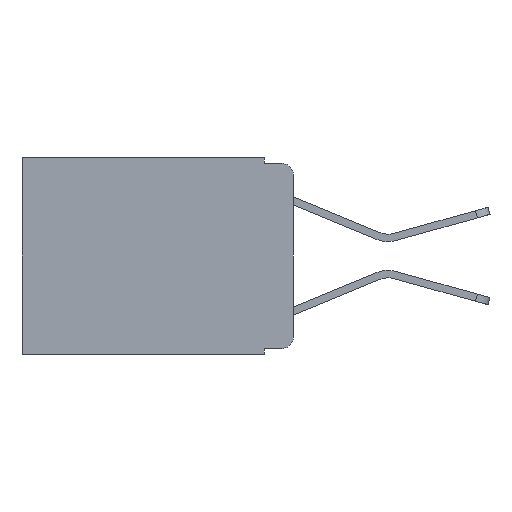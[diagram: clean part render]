
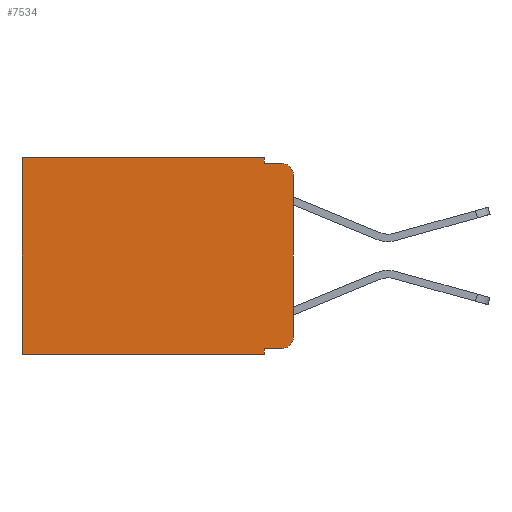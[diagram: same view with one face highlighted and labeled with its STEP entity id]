
A CAD part, left-side view. The second image highlights one B-rep face of the part: STEP entity #7534.
In plain terms, the highlighted planar face has unit normal (-1, 0, 0).
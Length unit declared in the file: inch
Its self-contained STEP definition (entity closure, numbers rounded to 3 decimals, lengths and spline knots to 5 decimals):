
#37 = DIRECTION ( 'NONE',  ( 0., 1., 0. ) ) ;
#145 = PLANE ( 'NONE',  #11362 ) ;
#223 = CARTESIAN_POINT ( 'NONE',  ( 0.298, 0.051, -0.333 ) ) ;
#269 = VERTEX_POINT ( 'NONE', #6955 ) ;
#425 = CARTESIAN_POINT ( 'NONE',  ( 0.298, 0.051, 0. ) ) ;
#492 = VERTEX_POINT ( 'NONE', #12710 ) ;
#496 = VERTEX_POINT ( 'NONE', #12790 ) ;
#734 = VECTOR ( 'NONE', #9410, 39.37008 ) ;
#867 = ORIENTED_EDGE ( 'NONE', *, *, #4749, .T. ) ;
#1336 = LINE ( 'NONE', #6577, #9643 ) ;
#1829 = DIRECTION ( 'NONE',  ( 0., 0., -1. ) ) ;
#1832 = CIRCLE ( 'NONE', #12632, 0.02 ) ;
#1895 = VERTEX_POINT ( 'NONE', #7905 ) ;
#1909 = VERTEX_POINT ( 'NONE', #4972 ) ;
#1985 = DIRECTION ( 'NONE',  ( 0., 0., -1. ) ) ;
#2217 = EDGE_CURVE ( 'NONE', #269, #6151, #1832, .T. ) ;
#2227 = ORIENTED_EDGE ( 'NONE', *, *, #4703, .F. ) ;
#2399 = EDGE_CURVE ( 'NONE', #11240, #269, #12608, .T. ) ;
#2665 = DIRECTION ( 'NONE',  ( 0., 0., -1. ) ) ;
#2772 = CARTESIAN_POINT ( 'NONE',  ( 0.298, 0., -0.03 ) ) ;
#3030 = CARTESIAN_POINT ( 'NONE',  ( 0.298, 0.051, -0.01 ) ) ;
#3244 = CIRCLE ( 'NONE', #12895, 0.02 ) ;
#4007 = ORIENTED_EDGE ( 'NONE', *, *, #4654, .F. ) ;
#4210 = DIRECTION ( 'NONE',  ( 0., -1., 0. ) ) ;
#4489 = LINE ( 'NONE', #11595, #9788 ) ;
#4553 = EDGE_CURVE ( 'NONE', #7193, #6151, #9804, .T. ) ;
#4568 = ORIENTED_EDGE ( 'NONE', *, *, #4945, .F. ) ;
#4598 = EDGE_CURVE ( 'NONE', #7193, #492, #3244, .T. ) ;
#4654 = EDGE_CURVE ( 'NONE', #12788, #496, #10535, .T. ) ;
#4683 = EDGE_CURVE ( 'NONE', #496, #492, #4925, .T. ) ;
#4703 = EDGE_CURVE ( 'NONE', #11240, #1909, #1336, .T. ) ;
#4749 = EDGE_CURVE ( 'NONE', #1895, #7877, #13625, .T. ) ;
#4925 = LINE ( 'NONE', #3030, #7258 ) ;
#4945 = EDGE_CURVE ( 'NONE', #1909, #7877, #12949, .T. ) ;
#4972 = CARTESIAN_POINT ( 'NONE',  ( 0.298, 0.051, -0.343 ) ) ;
#5606 = CARTESIAN_POINT ( 'NONE',  ( 0.298, 0., -0.313 ) ) ;
#5693 = DIRECTION ( 'NONE',  ( 0., -1., 0. ) ) ;
#6151 = VERTEX_POINT ( 'NONE', #5606 ) ;
#6332 = CARTESIAN_POINT ( 'NONE',  ( 0.298, 0.473, -0.343 ) ) ;
#6380 = CARTESIAN_POINT ( 'NONE',  ( 0.298, 0.02, -0.03 ) ) ;
#6477 = DIRECTION ( 'NONE',  ( 0., 0., -1. ) ) ;
#6572 = EDGE_CURVE ( 'NONE', #12788, #1895, #4489, .T. ) ;
#6577 = CARTESIAN_POINT ( 'NONE',  ( 0.298, 0.051, 0. ) ) ;
#6607 = CARTESIAN_POINT ( 'NONE',  ( 0.298, 0.02, -0.313 ) ) ;
#6955 = CARTESIAN_POINT ( 'NONE',  ( 0.298, 0.02, -0.333 ) ) ;
#7091 = ORIENTED_EDGE ( 'NONE', *, *, #2399, .T. ) ;
#7142 = VECTOR ( 'NONE', #5693, 39.37008 ) ;
#7193 = VERTEX_POINT ( 'NONE', #2772 ) ;
#7258 = VECTOR ( 'NONE', #4210, 39.37008 ) ;
#7528 = DIRECTION ( 'NONE',  ( 0., 0., -1. ) ) ;
#7534 = ADVANCED_FACE ( 'NONE', ( #12507 ), #145, .F. ) ;
#7806 = CARTESIAN_POINT ( 'NONE',  ( 0.298, 0.473, 0. ) ) ;
#7874 = ORIENTED_EDGE ( 'NONE', *, *, #6572, .T. ) ;
#7877 = VERTEX_POINT ( 'NONE', #6332 ) ;
#7905 = CARTESIAN_POINT ( 'NONE',  ( 0.298, 0.473, 0. ) ) ;
#7939 = VECTOR ( 'NONE', #6477, 39.37008 ) ;
#9038 = VECTOR ( 'NONE', #1985, 39.37008 ) ;
#9357 = DIRECTION ( 'NONE',  ( 1., 0., 0. ) ) ;
#9410 = DIRECTION ( 'NONE',  ( 0., 0., -1. ) ) ;
#9489 = ORIENTED_EDGE ( 'NONE', *, *, #4598, .T. ) ;
#9643 = VECTOR ( 'NONE', #1829, 39.37008 ) ;
#9707 = EDGE_LOOP ( 'NONE', ( #13335, #9489, #12260, #4007, #7874, #867, #4568, #2227, #7091, #12366 ) ) ;
#9788 = VECTOR ( 'NONE', #12533, 39.37008 ) ;
#9804 = LINE ( 'NONE', #10371, #734 ) ;
#10222 = VECTOR ( 'NONE', #37, 39.37008 ) ;
#10371 = CARTESIAN_POINT ( 'NONE',  ( 0.298, 0., 0. ) ) ;
#10425 = CARTESIAN_POINT ( 'NONE',  ( 0.298, 0.051, -0.333 ) ) ;
#10535 = LINE ( 'NONE', #10539, #7939 ) ;
#10539 = CARTESIAN_POINT ( 'NONE',  ( 0.298, 0.051, 0. ) ) ;
#11240 = VERTEX_POINT ( 'NONE', #223 ) ;
#11362 = AXIS2_PLACEMENT_3D ( 'NONE', #13042, #9357, #2665 ) ;
#11595 = CARTESIAN_POINT ( 'NONE',  ( 0.298, 0., 0. ) ) ;
#12260 = ORIENTED_EDGE ( 'NONE', *, *, #4683, .F. ) ;
#12366 = ORIENTED_EDGE ( 'NONE', *, *, #2217, .T. ) ;
#12507 = FACE_OUTER_BOUND ( 'NONE', #9707, .T. ) ;
#12533 = DIRECTION ( 'NONE',  ( 0., 1., 0. ) ) ;
#12608 = LINE ( 'NONE', #10425, #7142 ) ;
#12632 = AXIS2_PLACEMENT_3D ( 'NONE', #6607, #13378, #13484 ) ;
#12710 = CARTESIAN_POINT ( 'NONE',  ( 0.298, 0.02, -0.01 ) ) ;
#12788 = VERTEX_POINT ( 'NONE', #425 ) ;
#12790 = CARTESIAN_POINT ( 'NONE',  ( 0.298, 0.051, -0.01 ) ) ;
#12895 = AXIS2_PLACEMENT_3D ( 'NONE', #6380, #13208, #7528 ) ;
#12949 = LINE ( 'NONE', #13788, #10222 ) ;
#13042 = CARTESIAN_POINT ( 'NONE',  ( 0.298, 0., 0. ) ) ;
#13208 = DIRECTION ( 'NONE',  ( -1., 0., 0. ) ) ;
#13335 = ORIENTED_EDGE ( 'NONE', *, *, #4553, .F. ) ;
#13378 = DIRECTION ( 'NONE',  ( -1., 0., 0. ) ) ;
#13484 = DIRECTION ( 'NONE',  ( 0., 0., -1. ) ) ;
#13625 = LINE ( 'NONE', #7806, #9038 ) ;
#13788 = CARTESIAN_POINT ( 'NONE',  ( 0.298, 0., -0.343 ) ) ;
